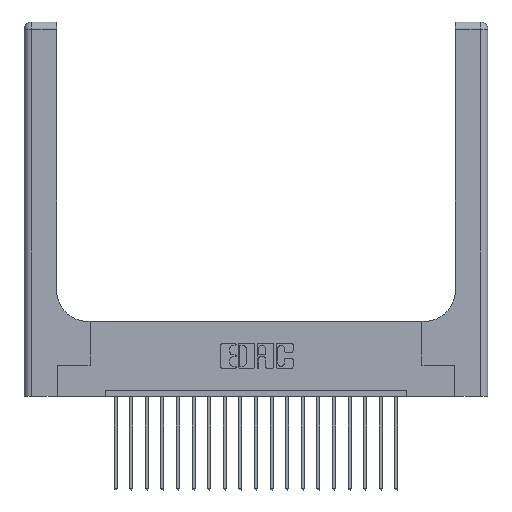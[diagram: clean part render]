
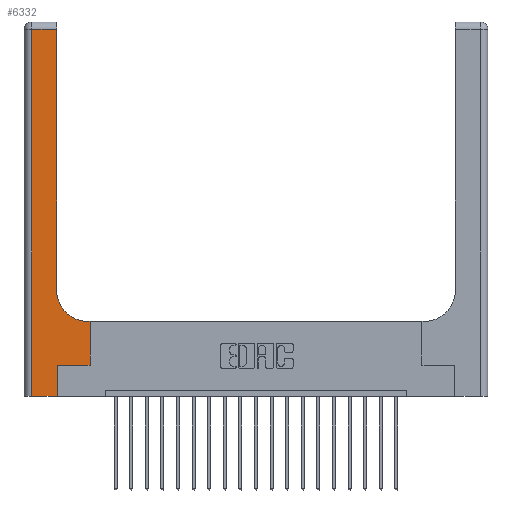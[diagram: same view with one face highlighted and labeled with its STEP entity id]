
A CAD part, top view. The second image highlights one B-rep face of the part: STEP entity #6332.
In plain terms, the highlighted planar face has unit normal (0, 0, 1).
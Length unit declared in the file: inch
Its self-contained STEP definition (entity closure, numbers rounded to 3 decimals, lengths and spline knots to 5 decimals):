
#27 = ORIENTED_EDGE ( 'NONE', *, *, #13184, .T. ) ;
#60 = VECTOR ( 'NONE', #6219, 39.37008 ) ;
#601 = CARTESIAN_POINT ( 'NONE',  ( 0.265, 0., 0.37 ) ) ;
#771 = LINE ( 'NONE', #13472, #12646 ) ;
#805 = LINE ( 'NONE', #5297, #15350 ) ;
#895 = EDGE_LOOP ( 'NONE', ( #16085, #13675, #2301, #7319, #12995, #19782, #3690, #27, #17809 ) ) ;
#925 = VERTEX_POINT ( 'NONE', #11126 ) ;
#1527 = VECTOR ( 'NONE', #12205, 39.37008 ) ;
#2190 = DIRECTION ( 'NONE',  ( 1., 0., 0. ) ) ;
#2301 = ORIENTED_EDGE ( 'NONE', *, *, #19090, .T. ) ;
#2604 = VERTEX_POINT ( 'NONE', #5028 ) ;
#2831 = AXIS2_PLACEMENT_3D ( 'NONE', #13407, #11784, #14779 ) ;
#3068 = EDGE_CURVE ( 'NONE', #19857, #925, #8302, .T. ) ;
#3070 = VERTEX_POINT ( 'NONE', #11292 ) ;
#3244 = VERTEX_POINT ( 'NONE', #13428 ) ;
#3690 = ORIENTED_EDGE ( 'NONE', *, *, #5443, .T. ) ;
#3873 = VECTOR ( 'NONE', #16780, 39.37008 ) ;
#3899 = VECTOR ( 'NONE', #13629, 39.37008 ) ;
#4268 = EDGE_CURVE ( 'NONE', #19925, #2604, #771, .T. ) ;
#4729 = LINE ( 'NONE', #12415, #60 ) ;
#5028 = CARTESIAN_POINT ( 'NONE',  ( 0.528, 0.25, 0.37 ) ) ;
#5297 = CARTESIAN_POINT ( 'NONE',  ( 0., 0., 0.37 ) ) ;
#5386 = VECTOR ( 'NONE', #14486, 39.37008 ) ;
#5443 = EDGE_CURVE ( 'NONE', #2604, #18569, #7762, .T. ) ;
#5551 = LINE ( 'NONE', #10525, #3873 ) ;
#5992 = CARTESIAN_POINT ( 'NONE',  ( 0., 3., 0.37 ) ) ;
#6219 = DIRECTION ( 'NONE',  ( -1., 0., 0. ) ) ;
#6332 = ADVANCED_FACE ( 'NONE', ( #10106 ), #18241, .F. ) ;
#6450 = CARTESIAN_POINT ( 'NONE',  ( 0., 2.94, 0.37 ) ) ;
#7319 = ORIENTED_EDGE ( 'NONE', *, *, #15493, .T. ) ;
#7762 = LINE ( 'NONE', #19526, #3899 ) ;
#8049 = LINE ( 'NONE', #601, #5386 ) ;
#8101 = LINE ( 'NONE', #16768, #1527 ) ;
#8302 = LINE ( 'NONE', #6450, #10247 ) ;
#8405 = CARTESIAN_POINT ( 'NONE',  ( 0.26, 2.94, 0.37 ) ) ;
#8983 = CARTESIAN_POINT ( 'NONE',  ( 0.265, 0.25, 0.37 ) ) ;
#9027 = DIRECTION ( 'NONE',  ( 0., 0., -1. ) ) ;
#9614 = DIRECTION ( 'NONE',  ( -1., 0., 0. ) ) ;
#10106 = FACE_OUTER_BOUND ( 'NONE', #895, .T. ) ;
#10174 = CARTESIAN_POINT ( 'NONE',  ( 0.51, 0.6, 0.37 ) ) ;
#10247 = VECTOR ( 'NONE', #9614, 39.37008 ) ;
#10525 = CARTESIAN_POINT ( 'NONE',  ( 0.06, 3., 0.37 ) ) ;
#11126 = CARTESIAN_POINT ( 'NONE',  ( 0.06, 2.94, 0.37 ) ) ;
#11292 = CARTESIAN_POINT ( 'NONE',  ( 0.06, 0., 0.37 ) ) ;
#11643 = DIRECTION ( 'NONE',  ( 1., 0., 0. ) ) ;
#11784 = DIRECTION ( 'NONE',  ( 0., 0., -1. ) ) ;
#12205 = DIRECTION ( 'NONE',  ( 0., 1., 0. ) ) ;
#12415 = CARTESIAN_POINT ( 'NONE',  ( 0.26, 0.6, 0.37 ) ) ;
#12421 = CARTESIAN_POINT ( 'NONE',  ( 0.265, 0., 0.37 ) ) ;
#12643 = CARTESIAN_POINT ( 'NONE',  ( 0.528, 0.6, 0.37 ) ) ;
#12646 = VECTOR ( 'NONE', #11643, 39.37008 ) ;
#12995 = ORIENTED_EDGE ( 'NONE', *, *, #16408, .T. ) ;
#13184 = EDGE_CURVE ( 'NONE', #18569, #14597, #4729, .T. ) ;
#13407 = CARTESIAN_POINT ( 'NONE',  ( 0.51, 0.85, 0.37 ) ) ;
#13428 = CARTESIAN_POINT ( 'NONE',  ( 0.26, 0.85, 0.37 ) ) ;
#13472 = CARTESIAN_POINT ( 'NONE',  ( 0.265, 0.25, 0.37 ) ) ;
#13629 = DIRECTION ( 'NONE',  ( 0., 1., 0. ) ) ;
#13675 = ORIENTED_EDGE ( 'NONE', *, *, #3068, .T. ) ;
#13800 = EDGE_CURVE ( 'NONE', #3244, #19857, #8101, .T. ) ;
#14486 = DIRECTION ( 'NONE',  ( 0., 1., 0. ) ) ;
#14597 = VERTEX_POINT ( 'NONE', #10174 ) ;
#14779 = DIRECTION ( 'NONE',  ( 1., 0., 0. ) ) ;
#15116 = DIRECTION ( 'NONE',  ( -1., 0., 0. ) ) ;
#15350 = VECTOR ( 'NONE', #2190, 39.37008 ) ;
#15493 = EDGE_CURVE ( 'NONE', #3070, #17323, #805, .T. ) ;
#16085 = ORIENTED_EDGE ( 'NONE', *, *, #13800, .T. ) ;
#16408 = EDGE_CURVE ( 'NONE', #17323, #19925, #8049, .T. ) ;
#16768 = CARTESIAN_POINT ( 'NONE',  ( 0.26, 3., 0.37 ) ) ;
#16780 = DIRECTION ( 'NONE',  ( 0., -1., 0. ) ) ;
#17323 = VERTEX_POINT ( 'NONE', #12421 ) ;
#17723 = EDGE_CURVE ( 'NONE', #14597, #3244, #19611, .T. ) ;
#17809 = ORIENTED_EDGE ( 'NONE', *, *, #17723, .T. ) ;
#18238 = AXIS2_PLACEMENT_3D ( 'NONE', #5992, #9027, #15116 ) ;
#18241 = PLANE ( 'NONE',  #18238 ) ;
#18569 = VERTEX_POINT ( 'NONE', #12643 ) ;
#19090 = EDGE_CURVE ( 'NONE', #925, #3070, #5551, .T. ) ;
#19526 = CARTESIAN_POINT ( 'NONE',  ( 0.528, 0.25, 0.37 ) ) ;
#19611 = CIRCLE ( 'NONE', #2831, 0.25 ) ;
#19782 = ORIENTED_EDGE ( 'NONE', *, *, #4268, .T. ) ;
#19857 = VERTEX_POINT ( 'NONE', #8405 ) ;
#19925 = VERTEX_POINT ( 'NONE', #8983 ) ;
